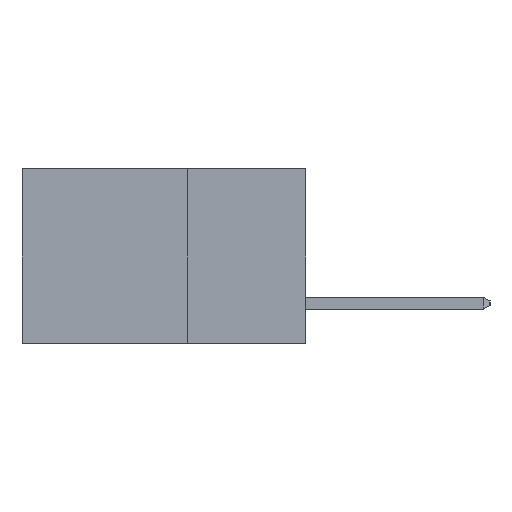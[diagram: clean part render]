
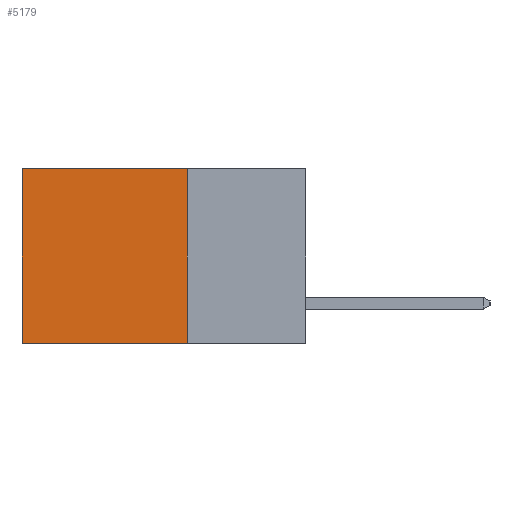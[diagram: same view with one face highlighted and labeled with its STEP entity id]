
A CAD part, left-side view. The second image highlights one B-rep face of the part: STEP entity #5179.
In plain terms, the highlighted planar face has unit normal (-1, 0, 0).
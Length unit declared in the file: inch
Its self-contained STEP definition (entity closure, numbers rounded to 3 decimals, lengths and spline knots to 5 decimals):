
#876 = CARTESIAN_POINT ( 'NONE',  ( 0.2615, 0.25, -0.37 ) ) ;
#922 = DIRECTION ( 'NONE',  ( 0., 1., 0. ) ) ;
#1107 = VERTEX_POINT ( 'NONE', #11233 ) ;
#1542 = PLANE ( 'NONE',  #2371 ) ;
#1639 = DIRECTION ( 'NONE',  ( 0., 1., 0. ) ) ;
#1655 = EDGE_LOOP ( 'NONE', ( #9547, #9845, #10150, #10441 ) ) ;
#1941 = FACE_OUTER_BOUND ( 'NONE', #1655, .T. ) ;
#2371 = AXIS2_PLACEMENT_3D ( 'NONE', #10122, #8227, #2494 ) ;
#2388 = EDGE_CURVE ( 'NONE', #3762, #11757, #2466, .T. ) ;
#2466 = LINE ( 'NONE', #876, #7604 ) ;
#2494 = DIRECTION ( 'NONE',  ( 0., 0., -1. ) ) ;
#2788 = VERTEX_POINT ( 'NONE', #5571 ) ;
#3119 = DIRECTION ( 'NONE',  ( 0., 0., -1. ) ) ;
#3233 = CARTESIAN_POINT ( 'NONE',  ( 0.2615, 0.6, -0.37 ) ) ;
#3480 = CARTESIAN_POINT ( 'NONE',  ( 0.2615, 0.6, -0.37 ) ) ;
#3762 = VERTEX_POINT ( 'NONE', #9078 ) ;
#4047 = EDGE_CURVE ( 'NONE', #1107, #11757, #11822, .T. ) ;
#5179 = ADVANCED_FACE ( 'NONE', ( #1941 ), #1542, .F. ) ;
#5312 = CARTESIAN_POINT ( 'NONE',  ( 0.2615, 0.25, -0.37 ) ) ;
#5571 = CARTESIAN_POINT ( 'NONE',  ( 0.2615, 0.25, 0. ) ) ;
#5799 = LINE ( 'NONE', #7655, #10497 ) ;
#6907 = EDGE_CURVE ( 'NONE', #2788, #3762, #12075, .T. ) ;
#7604 = VECTOR ( 'NONE', #1639, 39.37008 ) ;
#7655 = CARTESIAN_POINT ( 'NONE',  ( 0.2615, 0.25, 0. ) ) ;
#8227 = DIRECTION ( 'NONE',  ( 1., 0., 0. ) ) ;
#9064 = DIRECTION ( 'NONE',  ( 0., 0., -1. ) ) ;
#9078 = CARTESIAN_POINT ( 'NONE',  ( 0.2615, 0.25, -0.37 ) ) ;
#9179 = EDGE_CURVE ( 'NONE', #2788, #1107, #5799, .T. ) ;
#9323 = VECTOR ( 'NONE', #3119, 39.37008 ) ;
#9547 = ORIENTED_EDGE ( 'NONE', *, *, #4047, .T. ) ;
#9567 = VECTOR ( 'NONE', #9064, 39.37008 ) ;
#9845 = ORIENTED_EDGE ( 'NONE', *, *, #2388, .F. ) ;
#10122 = CARTESIAN_POINT ( 'NONE',  ( 0.2615, 0.25, -0.37 ) ) ;
#10150 = ORIENTED_EDGE ( 'NONE', *, *, #6907, .F. ) ;
#10441 = ORIENTED_EDGE ( 'NONE', *, *, #9179, .T. ) ;
#10497 = VECTOR ( 'NONE', #922, 39.37008 ) ;
#11233 = CARTESIAN_POINT ( 'NONE',  ( 0.2615, 0.6, 0. ) ) ;
#11757 = VERTEX_POINT ( 'NONE', #3480 ) ;
#11822 = LINE ( 'NONE', #3233, #9323 ) ;
#12075 = LINE ( 'NONE', #5312, #9567 ) ;
